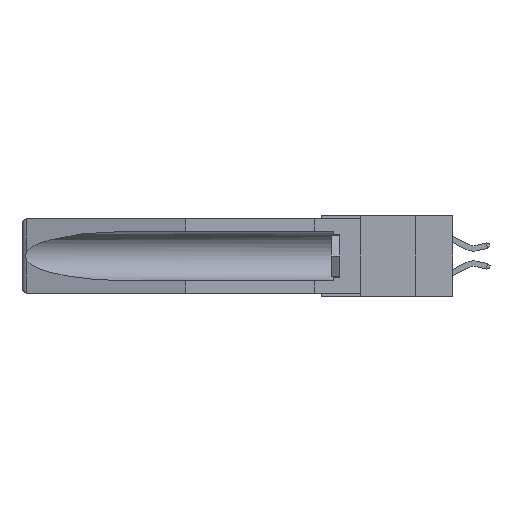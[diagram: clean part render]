
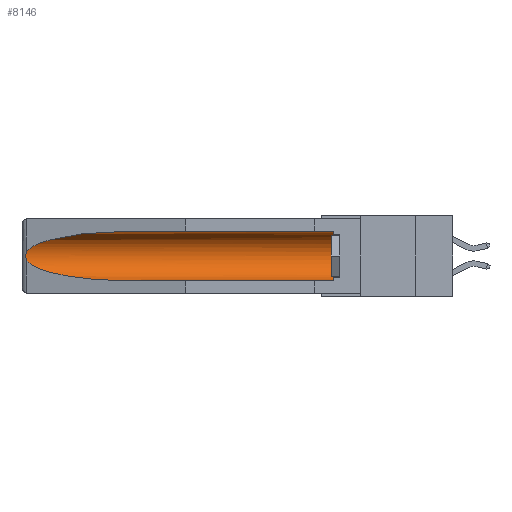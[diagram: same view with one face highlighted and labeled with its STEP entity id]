
A CAD part, left-side view. The second image highlights one B-rep face of the part: STEP entity #8146.
In plain terms, the highlighted cylindrical face has radius 2.857 mm (diameter 5.715 mm), a partial arc.
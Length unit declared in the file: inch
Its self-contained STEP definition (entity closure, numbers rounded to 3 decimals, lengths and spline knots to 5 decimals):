
#247 = EDGE_CURVE ( 'NONE', #13077, #11645, #7923, .T. ) ;
#1029 = VERTEX_POINT ( 'NONE', #13038 ) ;
#2069 = CARTESIAN_POINT ( 'NONE',  ( 0.155, 1.07973, -0.284 ) ) ;
#3272 = CARTESIAN_POINT ( 'NONE',  ( 0.26537, 1.52718, -0.14972 ) ) ;
#3746 = CARTESIAN_POINT ( 'NONE',  ( 0.2673, 1.53269, -0.17917 ) ) ;
#3991 = CARTESIAN_POINT ( 'NONE',  ( 0.155, 1.07973, -0.059 ) ) ;
#4078 = CARTESIAN_POINT ( 'NONE',  ( 0.25451, 1.48313, -0.24835 ) ) ;
#4099 = CARTESIAN_POINT ( 'NONE',  ( 0.155, 1.07973, -0.059 ) ) ;
#4221 = EDGE_CURVE ( 'NONE', #1029, #21220, #6859, .T. ) ;
#4756 = EDGE_LOOP ( 'NONE', ( #27542, #19698, #13098, #25247, #25125, #5362 ) ) ;
#4998 = CARTESIAN_POINT ( 'NONE',  ( 0.26537, 1.52718, -0.19328 ) ) ;
#5362 = ORIENTED_EDGE ( 'NONE', *, *, #26002, .T. ) ;
#5639 = CARTESIAN_POINT ( 'NONE',  ( 0.26597, 1.52961, -0.15275 ) ) ;
#6010 = CARTESIAN_POINT ( 'NONE',  ( 0.26655, 1.53094, -0.18657 ) ) ;
#6331 = CARTESIAN_POINT ( 'NONE',  ( 0.21114, 1.30732, -0.284 ) ) ;
#6859 = CIRCLE ( 'NONE', #23423, 0.1125 ) ;
#7156 = VERTEX_POINT ( 'NONE', #3991 ) ;
#7923 =( BOUNDED_CURVE ( )  B_SPLINE_CURVE ( 3, ( #10819, #4078, #6331, #2069 ),
 .UNSPECIFIED., .F., .F. ) 
 B_SPLINE_CURVE_WITH_KNOTS ( ( 4, 4 ),
 ( 0.1948, 1.5708 ),
 .UNSPECIFIED. ) 
 CURVE ( )  GEOMETRIC_REPRESENTATION_ITEM ( )  RATIONAL_B_SPLINE_CURVE ( ( 1., 0.848, 0.848, 1. ) ) 
 REPRESENTATION_ITEM ( '' )  );
#8146 = ADVANCED_FACE ( 'NONE', ( #24397 ), #12800, .F. ) ;
#8857 = CARTESIAN_POINT ( 'NONE',  ( 0.155, -0.30754, -0.1715 ) ) ;
#8965 = VERTEX_POINT ( 'NONE', #20115 ) ;
#9036 = VECTOR ( 'NONE', #9550, 39.37008 ) ;
#9550 = DIRECTION ( 'NONE',  ( 0., 1., 0. ) ) ;
#9554 = CARTESIAN_POINT ( 'NONE',  ( 0.155, 0.126, -0.059 ) ) ;
#10044 = CARTESIAN_POINT ( 'NONE',  ( 0.155, 1.07973, -0.284 ) ) ;
#10378 = CARTESIAN_POINT ( 'NONE',  ( 0.155, 0.126, -0.1715 ) ) ;
#10819 = CARTESIAN_POINT ( 'NONE',  ( 0.26537, 1.52718, -0.19328 ) ) ;
#11014 = EDGE_CURVE ( 'NONE', #8965, #13077, #20744, .T. ) ;
#11645 = VERTEX_POINT ( 'NONE', #10044 ) ;
#11776 = LINE ( 'NONE', #24753, #9036 ) ;
#12800 = CYLINDRICAL_SURFACE ( 'NONE', #25144, 0.1125 ) ;
#13027 = EDGE_CURVE ( 'NONE', #1029, #11645, #26228, .T. ) ;
#13038 = CARTESIAN_POINT ( 'NONE',  ( 0.155, 0.126, -0.284 ) ) ;
#13077 = VERTEX_POINT ( 'NONE', #4998 ) ;
#13098 = ORIENTED_EDGE ( 'NONE', *, *, #247, .T. ) ;
#13559 = DIRECTION ( 'NONE',  ( 0., 0., 1. ) ) ;
#14641 = CARTESIAN_POINT ( 'NONE',  ( 0.2675, 1.53308, -0.16763 ) ) ;
#14737 = CARTESIAN_POINT ( 'NONE',  ( 0.2675, 1.53308, -0.17534 ) ) ;
#15177 = CARTESIAN_POINT ( 'NONE',  ( 0.21114, 1.30732, -0.059 ) ) ;
#15348 = DIRECTION ( 'NONE',  ( 0., 1., 0. ) ) ;
#15654 =( BOUNDED_CURVE ( )  B_SPLINE_CURVE ( 3, ( #4099, #15177, #21507, #26137 ),
 .UNSPECIFIED., .F., .F. ) 
 B_SPLINE_CURVE_WITH_KNOTS ( ( 4, 4 ),
 ( 4.71239, 6.08839 ),
 .UNSPECIFIED. ) 
 CURVE ( )  GEOMETRIC_REPRESENTATION_ITEM ( )  RATIONAL_B_SPLINE_CURVE ( ( 1., 0.848, 0.848, 1. ) ) 
 REPRESENTATION_ITEM ( '' )  );
#19134 = CARTESIAN_POINT ( 'NONE',  ( 0.2673, 1.5327, -0.16383 ) ) ;
#19291 = DIRECTION ( 'NONE',  ( 0., -1., 0. ) ) ;
#19698 = ORIENTED_EDGE ( 'NONE', *, *, #11014, .T. ) ;
#20115 = CARTESIAN_POINT ( 'NONE',  ( 0.26537, 1.52718, -0.14972 ) ) ;
#20274 = DIRECTION ( 'NONE',  ( 0., 1., 0. ) ) ;
#20744 = B_SPLINE_CURVE_WITH_KNOTS ( 'NONE', 3,
 ( #3272, #5639, #25513, #19134, #14641, #14737, #3746, #6010, #26160, #28090 ),
 .UNSPECIFIED., .F., .F.,
 ( 4, 2, 2, 2, 4 ),
 ( 0., 0.00029, 0.00058, 0.00087, 0.00117 ),
 .UNSPECIFIED. ) ;
#21220 = VERTEX_POINT ( 'NONE', #9554 ) ;
#21507 = CARTESIAN_POINT ( 'NONE',  ( 0.25451, 1.48313, -0.09465 ) ) ;
#23423 = AXIS2_PLACEMENT_3D ( 'NONE', #10378, #19291, #27867 ) ;
#24397 = FACE_OUTER_BOUND ( 'NONE', #4756, .T. ) ;
#24753 = CARTESIAN_POINT ( 'NONE',  ( 0.155, -0.30754, -0.059 ) ) ;
#25125 = ORIENTED_EDGE ( 'NONE', *, *, #4221, .T. ) ;
#25144 = AXIS2_PLACEMENT_3D ( 'NONE', #8857, #20274, #13559 ) ;
#25239 = VECTOR ( 'NONE', #15348, 39.37008 ) ;
#25247 = ORIENTED_EDGE ( 'NONE', *, *, #13027, .F. ) ;
#25513 = CARTESIAN_POINT ( 'NONE',  ( 0.26654, 1.53092, -0.15636 ) ) ;
#26002 = EDGE_CURVE ( 'NONE', #21220, #7156, #11776, .T. ) ;
#26137 = CARTESIAN_POINT ( 'NONE',  ( 0.26537, 1.52718, -0.14972 ) ) ;
#26160 = CARTESIAN_POINT ( 'NONE',  ( 0.26597, 1.5296, -0.19026 ) ) ;
#26202 = EDGE_CURVE ( 'NONE', #7156, #8965, #15654, .T. ) ;
#26228 = LINE ( 'NONE', #26406, #25239 ) ;
#26406 = CARTESIAN_POINT ( 'NONE',  ( 0.155, -0.30754, -0.284 ) ) ;
#27542 = ORIENTED_EDGE ( 'NONE', *, *, #26202, .T. ) ;
#27867 = DIRECTION ( 'NONE',  ( 0., 0., 1. ) ) ;
#28090 = CARTESIAN_POINT ( 'NONE',  ( 0.26537, 1.52718, -0.19328 ) ) ;
